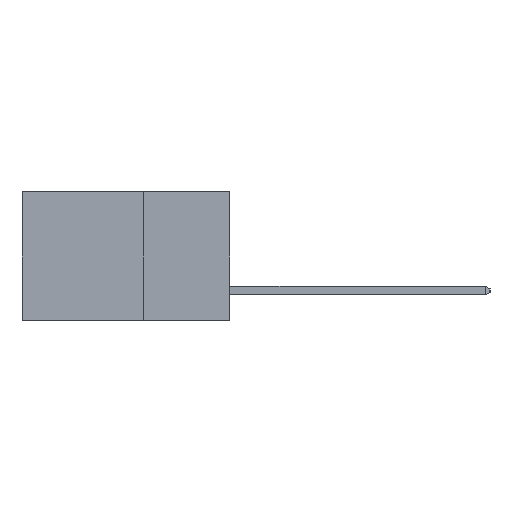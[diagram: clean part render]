
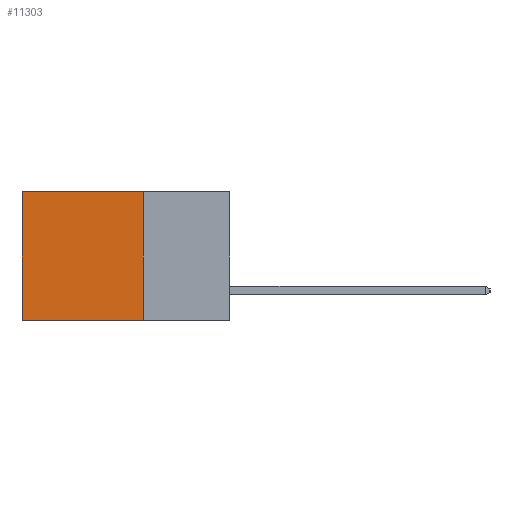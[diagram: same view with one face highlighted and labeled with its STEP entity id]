
A CAD part, left-side view. The second image highlights one B-rep face of the part: STEP entity #11303.
In plain terms, the highlighted planar face has unit normal (-1, 0, 0).
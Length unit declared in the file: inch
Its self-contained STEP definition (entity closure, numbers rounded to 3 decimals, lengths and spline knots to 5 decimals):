
#709 = CARTESIAN_POINT ( 'NONE',  ( 0.2615, 0.25, 0. ) ) ;
#724 = DIRECTION ( 'NONE',  ( 0., 1., 0. ) ) ;
#1604 = VERTEX_POINT ( 'NONE', #2291 ) ;
#1975 = ORIENTED_EDGE ( 'NONE', *, *, #2899, .T. ) ;
#2291 = CARTESIAN_POINT ( 'NONE',  ( 0.2615, 0.6, -0.37 ) ) ;
#2364 = ORIENTED_EDGE ( 'NONE', *, *, #2497, .F. ) ;
#2497 = EDGE_CURVE ( 'NONE', #13026, #10996, #8832, .T. ) ;
#2899 = EDGE_CURVE ( 'NONE', #13026, #12210, #7229, .T. ) ;
#3169 = EDGE_CURVE ( 'NONE', #10996, #1604, #9466, .T. ) ;
#3584 = DIRECTION ( 'NONE',  ( 0., 0., -1. ) ) ;
#4111 = CARTESIAN_POINT ( 'NONE',  ( 0.2615, 0.25, -0.37 ) ) ;
#4326 = FACE_OUTER_BOUND ( 'NONE', #7182, .T. ) ;
#4510 = ORIENTED_EDGE ( 'NONE', *, *, #11329, .T. ) ;
#4962 = CARTESIAN_POINT ( 'NONE',  ( 0.2615, 0.6, 0. ) ) ;
#5168 = AXIS2_PLACEMENT_3D ( 'NONE', #5621, #5670, #12835 ) ;
#5621 = CARTESIAN_POINT ( 'NONE',  ( 0.2615, 0.25, -0.37 ) ) ;
#5670 = DIRECTION ( 'NONE',  ( 1., 0., 0. ) ) ;
#5674 = DIRECTION ( 'NONE',  ( 0., 0., -1. ) ) ;
#5712 = CARTESIAN_POINT ( 'NONE',  ( 0.2615, 0.25, -0.37 ) ) ;
#6726 = VECTOR ( 'NONE', #11111, 39.37008 ) ;
#7182 = EDGE_LOOP ( 'NONE', ( #4510, #7299, #2364, #1975 ) ) ;
#7229 = LINE ( 'NONE', #709, #9967 ) ;
#7299 = ORIENTED_EDGE ( 'NONE', *, *, #3169, .F. ) ;
#7679 = PLANE ( 'NONE',  #5168 ) ;
#8528 = VECTOR ( 'NONE', #5674, 39.37008 ) ;
#8832 = LINE ( 'NONE', #5712, #8528 ) ;
#9046 = CARTESIAN_POINT ( 'NONE',  ( 0.2615, 0.25, -0.37 ) ) ;
#9466 = LINE ( 'NONE', #9046, #6726 ) ;
#9497 = LINE ( 'NONE', #11856, #11895 ) ;
#9967 = VECTOR ( 'NONE', #724, 39.37008 ) ;
#10996 = VERTEX_POINT ( 'NONE', #4111 ) ;
#11111 = DIRECTION ( 'NONE',  ( 0., 1., 0. ) ) ;
#11303 = ADVANCED_FACE ( 'NONE', ( #4326 ), #7679, .F. ) ;
#11329 = EDGE_CURVE ( 'NONE', #12210, #1604, #9497, .T. ) ;
#11593 = CARTESIAN_POINT ( 'NONE',  ( 0.2615, 0.25, 0. ) ) ;
#11856 = CARTESIAN_POINT ( 'NONE',  ( 0.2615, 0.6, -0.37 ) ) ;
#11895 = VECTOR ( 'NONE', #3584, 39.37008 ) ;
#12210 = VERTEX_POINT ( 'NONE', #4962 ) ;
#12835 = DIRECTION ( 'NONE',  ( 0., 0., -1. ) ) ;
#13026 = VERTEX_POINT ( 'NONE', #11593 ) ;
